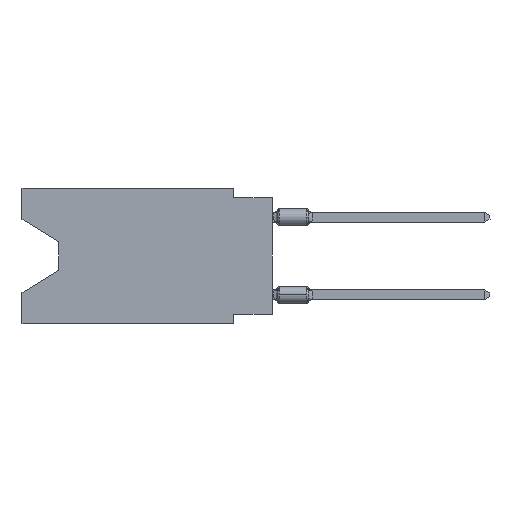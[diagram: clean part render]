
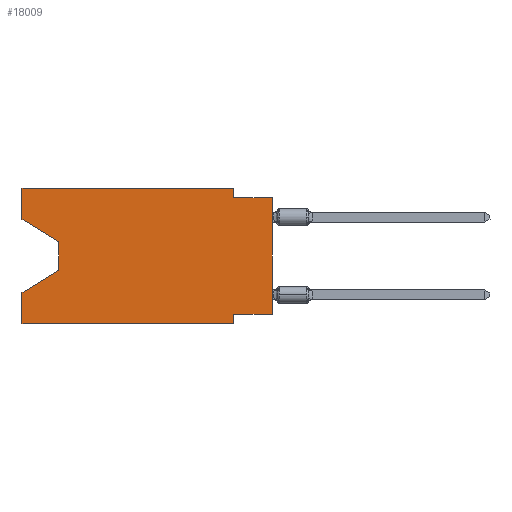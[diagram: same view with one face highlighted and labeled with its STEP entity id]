
A CAD part, left-side view. The second image highlights one B-rep face of the part: STEP entity #18009.
In plain terms, the highlighted planar face has unit normal (-1, 0, 0).
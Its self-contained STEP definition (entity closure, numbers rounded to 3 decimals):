
#598 = EDGE_CURVE ( 'NONE', #27207, #5002, #20628, .T. ) ;
#694 = CARTESIAN_POINT ( 'NONE',  ( 0., 0., -8.255 ) ) ;
#1076 = PLANE ( 'NONE',  #23325 ) ;
#1622 = ORIENTED_EDGE ( 'NONE', *, *, #21236, .T. ) ;
#2063 = ORIENTED_EDGE ( 'NONE', *, *, #10433, .F. ) ;
#2342 = CARTESIAN_POINT ( 'NONE',  ( 0., 16.383, 0. ) ) ;
#2700 = ORIENTED_EDGE ( 'NONE', *, *, #6132, .F. ) ;
#2705 = ORIENTED_EDGE ( 'NONE', *, *, #598, .F. ) ;
#3293 = ORIENTED_EDGE ( 'NONE', *, *, #7225, .F. ) ;
#3557 = DIRECTION ( 'NONE',  ( 1., 0., 0. ) ) ;
#3750 = VECTOR ( 'NONE', #19118, 1000. ) ;
#3894 = CARTESIAN_POINT ( 'NONE',  ( 0., 16.383, -8.89 ) ) ;
#4602 = VECTOR ( 'NONE', #24091, 1000. ) ;
#5002 = VERTEX_POINT ( 'NONE', #22216 ) ;
#5177 = CARTESIAN_POINT ( 'NONE',  ( 0., 13.97, -3.505 ) ) ;
#5533 = VECTOR ( 'NONE', #16245, 1000. ) ;
#5947 = CARTESIAN_POINT ( 'NONE',  ( 0., 2.54, 0. ) ) ;
#6132 = EDGE_CURVE ( 'NONE', #23738, #21079, #13275, .T. ) ;
#6468 = EDGE_CURVE ( 'NONE', #25793, #17873, #19406, .T. ) ;
#6874 = CARTESIAN_POINT ( 'NONE',  ( 0., 2.54, -8.255 ) ) ;
#6987 = DIRECTION ( 'NONE',  ( 0., 0., -1. ) ) ;
#7225 = EDGE_CURVE ( 'NONE', #22268, #23738, #7633, .T. ) ;
#7424 = VECTOR ( 'NONE', #22388, 1000. ) ;
#7556 = VECTOR ( 'NONE', #28760, 1000. ) ;
#7633 = LINE ( 'NONE', #25211, #10640 ) ;
#8121 = LINE ( 'NONE', #25871, #3750 ) ;
#8271 = VERTEX_POINT ( 'NONE', #12998 ) ;
#9687 = VERTEX_POINT ( 'NONE', #3894 ) ;
#10433 = EDGE_CURVE ( 'NONE', #26403, #27207, #25233, .T. ) ;
#10640 = VECTOR ( 'NONE', #16568, 1000. ) ;
#11174 = CARTESIAN_POINT ( 'NONE',  ( 0., 0., 0. ) ) ;
#11425 = EDGE_CURVE ( 'NONE', #26403, #8271, #15280, .T. ) ;
#11691 = CARTESIAN_POINT ( 'NONE',  ( 0., 16.383, -6.852 ) ) ;
#11858 = LINE ( 'NONE', #20361, #5533 ) ;
#12494 = DIRECTION ( 'NONE',  ( 0., 0., -1. ) ) ;
#12705 = DIRECTION ( 'NONE',  ( 0., 0., -1. ) ) ;
#12998 = CARTESIAN_POINT ( 'NONE',  ( 0., 0., -0.635 ) ) ;
#13122 = LINE ( 'NONE', #19863, #15222 ) ;
#13160 = LINE ( 'NONE', #17698, #7424 ) ;
#13275 = LINE ( 'NONE', #5947, #27542 ) ;
#13926 = ORIENTED_EDGE ( 'NONE', *, *, #6468, .T. ) ;
#13975 = CARTESIAN_POINT ( 'NONE',  ( 0., 13.97, -3.505 ) ) ;
#14697 = CARTESIAN_POINT ( 'NONE',  ( 0., 16.383, 0. ) ) ;
#14733 = EDGE_LOOP ( 'NONE', ( #13926, #22086, #28061, #25909, #1622, #2705, #2063, #19020, #17316, #2700, #3293, #16775 ) ) ;
#15222 = VECTOR ( 'NONE', #21920, 1000. ) ;
#15280 = LINE ( 'NONE', #11174, #7556 ) ;
#15832 = CARTESIAN_POINT ( 'NONE',  ( 0., 16.383, -2.038 ) ) ;
#16245 = DIRECTION ( 'NONE',  ( 0., -1., 0. ) ) ;
#16568 = DIRECTION ( 'NONE',  ( 0., -1., 0. ) ) ;
#16614 = DIRECTION ( 'NONE',  ( 0., 0., -1. ) ) ;
#16775 = ORIENTED_EDGE ( 'NONE', *, *, #24810, .F. ) ;
#17316 = ORIENTED_EDGE ( 'NONE', *, *, #26917, .F. ) ;
#17698 = CARTESIAN_POINT ( 'NONE',  ( 0., 16.383, 0. ) ) ;
#17873 = VERTEX_POINT ( 'NONE', #5177 ) ;
#18009 = ADVANCED_FACE ( 'NONE', ( #25845 ), #1076, .F. ) ;
#19020 = ORIENTED_EDGE ( 'NONE', *, *, #11425, .T. ) ;
#19118 = DIRECTION ( 'NONE',  ( 0., -1., 0. ) ) ;
#19203 = VECTOR ( 'NONE', #22615, 1000. ) ;
#19272 = CARTESIAN_POINT ( 'NONE',  ( 0., 16.383, -2.038 ) ) ;
#19406 = LINE ( 'NONE', #19272, #4602 ) ;
#19863 = CARTESIAN_POINT ( 'NONE',  ( 0., 13.97, -5.385 ) ) ;
#20361 = CARTESIAN_POINT ( 'NONE',  ( 0., 16.383, -8.89 ) ) ;
#20445 = EDGE_CURVE ( 'NONE', #17873, #28682, #20589, .T. ) ;
#20589 = LINE ( 'NONE', #13975, #23766 ) ;
#20628 = LINE ( 'NONE', #25012, #20700 ) ;
#20668 = LINE ( 'NONE', #27705, #28825 ) ;
#20700 = VECTOR ( 'NONE', #6987, 1000. ) ;
#21079 = VERTEX_POINT ( 'NONE', #24321 ) ;
#21236 = EDGE_CURVE ( 'NONE', #9687, #5002, #11858, .T. ) ;
#21920 = DIRECTION ( 'NONE',  ( 0., 0.855, -0.519 ) ) ;
#22086 = ORIENTED_EDGE ( 'NONE', *, *, #20445, .T. ) ;
#22216 = CARTESIAN_POINT ( 'NONE',  ( 0., 2.54, -8.89 ) ) ;
#22268 = VERTEX_POINT ( 'NONE', #2342 ) ;
#22388 = DIRECTION ( 'NONE',  ( 0., 0., 1. ) ) ;
#22615 = DIRECTION ( 'NONE',  ( 0., 1., 0. ) ) ;
#22727 = EDGE_CURVE ( 'NONE', #9687, #28851, #13160, .T. ) ;
#23325 = AXIS2_PLACEMENT_3D ( 'NONE', #14697, #3557, #12494 ) ;
#23738 = VERTEX_POINT ( 'NONE', #26022 ) ;
#23766 = VECTOR ( 'NONE', #16614, 1000. ) ;
#24091 = DIRECTION ( 'NONE',  ( 0., -0.855, -0.519 ) ) ;
#24150 = CARTESIAN_POINT ( 'NONE',  ( 0., 13.97, -5.385 ) ) ;
#24321 = CARTESIAN_POINT ( 'NONE',  ( 0., 2.54, -0.635 ) ) ;
#24810 = EDGE_CURVE ( 'NONE', #25793, #22268, #20668, .T. ) ;
#25012 = CARTESIAN_POINT ( 'NONE',  ( 0., 2.54, -8.89 ) ) ;
#25211 = CARTESIAN_POINT ( 'NONE',  ( 0., 16.383, 0. ) ) ;
#25233 = LINE ( 'NONE', #27157, #19203 ) ;
#25437 = EDGE_CURVE ( 'NONE', #28682, #28851, #13122, .T. ) ;
#25793 = VERTEX_POINT ( 'NONE', #15832 ) ;
#25845 = FACE_OUTER_BOUND ( 'NONE', #14733, .T. ) ;
#25871 = CARTESIAN_POINT ( 'NONE',  ( 0., 0., -0.635 ) ) ;
#25909 = ORIENTED_EDGE ( 'NONE', *, *, #22727, .F. ) ;
#26022 = CARTESIAN_POINT ( 'NONE',  ( 0., 2.54, 0. ) ) ;
#26403 = VERTEX_POINT ( 'NONE', #694 ) ;
#26917 = EDGE_CURVE ( 'NONE', #21079, #8271, #8121, .T. ) ;
#27157 = CARTESIAN_POINT ( 'NONE',  ( 0., 0., -8.255 ) ) ;
#27207 = VERTEX_POINT ( 'NONE', #6874 ) ;
#27268 = DIRECTION ( 'NONE',  ( 0., 0., 1. ) ) ;
#27542 = VECTOR ( 'NONE', #12705, 1000. ) ;
#27705 = CARTESIAN_POINT ( 'NONE',  ( 0., 16.383, 0. ) ) ;
#28061 = ORIENTED_EDGE ( 'NONE', *, *, #25437, .T. ) ;
#28682 = VERTEX_POINT ( 'NONE', #24150 ) ;
#28760 = DIRECTION ( 'NONE',  ( 0., 0., 1. ) ) ;
#28825 = VECTOR ( 'NONE', #27268, 1000. ) ;
#28851 = VERTEX_POINT ( 'NONE', #11691 ) ;
